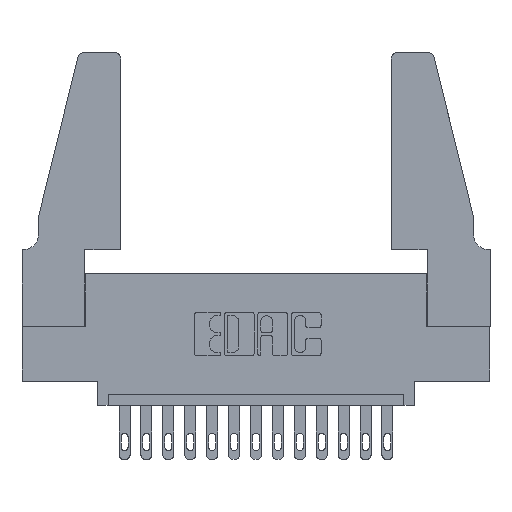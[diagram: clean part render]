
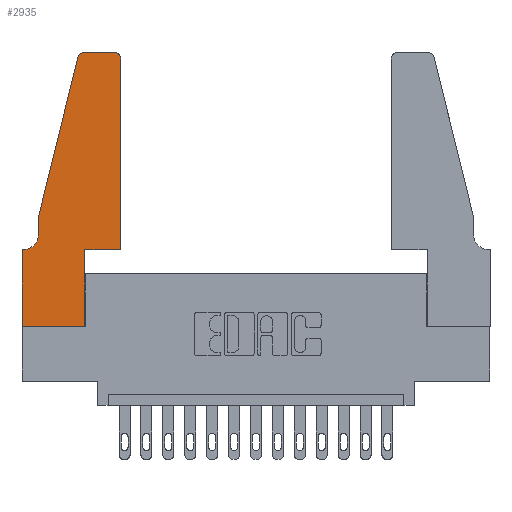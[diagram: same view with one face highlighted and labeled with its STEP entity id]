
A CAD part, top view. The second image highlights one B-rep face of the part: STEP entity #2935.
In plain terms, the highlighted planar face has unit normal (0, 0, 1).
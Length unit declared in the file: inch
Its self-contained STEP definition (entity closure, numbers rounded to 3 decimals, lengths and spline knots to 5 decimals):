
#66 = EDGE_CURVE ( 'NONE', #4315, #12217, #4490, .T. ) ;
#152 = CIRCLE ( 'NONE', #7703, 0.03 ) ;
#831 = CARTESIAN_POINT ( 'NONE',  ( 0.4505, 0.35, 0.37 ) ) ;
#885 = CARTESIAN_POINT ( 'NONE',  ( 0.0055, 0.42, 0.37 ) ) ;
#917 = EDGE_CURVE ( 'NONE', #12802, #11166, #6914, .T. ) ;
#943 = LINE ( 'NONE', #15656, #7222 ) ;
#964 = FACE_OUTER_BOUND ( 'NONE', #8152, .T. ) ;
#1023 = LINE ( 'NONE', #14323, #2944 ) ;
#1383 = CARTESIAN_POINT ( 'NONE',  ( 0.2865, 0., 0.37 ) ) ;
#1442 = CARTESIAN_POINT ( 'NONE',  ( 0.2865, 0.35, 0.37 ) ) ;
#1446 = VERTEX_POINT ( 'NONE', #4714 ) ;
#1695 = CARTESIAN_POINT ( 'NONE',  ( 0.0755, 0.35, 0.37 ) ) ;
#1713 = CARTESIAN_POINT ( 'NONE',  ( 0.0755, 0.5, 0.37 ) ) ;
#2155 = DIRECTION ( 'NONE',  ( 1., 0., 0. ) ) ;
#2235 = ORIENTED_EDGE ( 'NONE', *, *, #4029, .T. ) ;
#2286 = VECTOR ( 'NONE', #13903, 39.37008 ) ;
#2416 = ORIENTED_EDGE ( 'NONE', *, *, #11070, .T. ) ;
#2515 = CARTESIAN_POINT ( 'NONE',  ( 0.4505, 0.35, 0.37 ) ) ;
#2835 = VERTEX_POINT ( 'NONE', #6938 ) ;
#2844 = LINE ( 'NONE', #2515, #15338 ) ;
#2935 = ADVANCED_FACE ( 'NONE', ( #964 ), #7052, .T. ) ;
#2944 = VECTOR ( 'NONE', #10096, 39.37008 ) ;
#3166 = EDGE_CURVE ( 'NONE', #11661, #12802, #12251, .T. ) ;
#3444 = DIRECTION ( 'NONE',  ( 1., 0., 0. ) ) ;
#3966 = ORIENTED_EDGE ( 'NONE', *, *, #8165, .T. ) ;
#4029 = EDGE_CURVE ( 'NONE', #1446, #11661, #152, .T. ) ;
#4234 = DIRECTION ( 'NONE',  ( 0., -1., 0. ) ) ;
#4315 = VERTEX_POINT ( 'NONE', #15828 ) ;
#4490 = LINE ( 'NONE', #1695, #7522 ) ;
#4604 = VECTOR ( 'NONE', #14760, 39.37008 ) ;
#4714 = CARTESIAN_POINT ( 'NONE',  ( 0.4505, 1.22, 0.37 ) ) ;
#4883 = LINE ( 'NONE', #831, #9477 ) ;
#5033 = EDGE_CURVE ( 'NONE', #9683, #4315, #11062, .T. ) ;
#5145 = ORIENTED_EDGE ( 'NONE', *, *, #9306, .T. ) ;
#5272 = ORIENTED_EDGE ( 'NONE', *, *, #5033, .T. ) ;
#5331 = LINE ( 'NONE', #8982, #2286 ) ;
#5389 = ORIENTED_EDGE ( 'NONE', *, *, #66, .T. ) ;
#6042 = CARTESIAN_POINT ( 'NONE',  ( 0.4205, 1.22, 0.37 ) ) ;
#6242 = CARTESIAN_POINT ( 'NONE',  ( 0., 0., 0.37 ) ) ;
#6305 = ORIENTED_EDGE ( 'NONE', *, *, #8051, .T. ) ;
#6515 = DIRECTION ( 'NONE',  ( 1., 0., 0. ) ) ;
#6914 = CIRCLE ( 'NONE', #12190, 0.03 ) ;
#6938 = CARTESIAN_POINT ( 'NONE',  ( 0., 0., 0.37 ) ) ;
#7052 = PLANE ( 'NONE',  #7584 ) ;
#7111 = CARTESIAN_POINT ( 'NONE',  ( 0., 0.35, 0.37 ) ) ;
#7222 = VECTOR ( 'NONE', #4234, 39.37008 ) ;
#7522 = VECTOR ( 'NONE', #12796, 39.37008 ) ;
#7526 = EDGE_CURVE ( 'NONE', #2835, #10246, #10563, .T. ) ;
#7584 = AXIS2_PLACEMENT_3D ( 'NONE', #7111, #8141, #3444 ) ;
#7646 = EDGE_CURVE ( 'NONE', #10246, #10263, #5331, .T. ) ;
#7703 = AXIS2_PLACEMENT_3D ( 'NONE', #6042, #12357, #6515 ) ;
#8051 = EDGE_CURVE ( 'NONE', #12217, #2835, #943, .T. ) ;
#8141 = DIRECTION ( 'NONE',  ( 0., 0., 1. ) ) ;
#8152 = EDGE_LOOP ( 'NONE', ( #9585, #10078, #5145, #9146, #5272, #5389, #6305, #11058, #9573, #2416, #3966, #2235 ) ) ;
#8165 = EDGE_CURVE ( 'NONE', #8953, #1446, #2844, .T. ) ;
#8284 = DIRECTION ( 'NONE',  ( -0.239, -0.971, 0. ) ) ;
#8731 = CARTESIAN_POINT ( 'NONE',  ( 0.25487, 1.22718, 0.37 ) ) ;
#8922 = AXIS2_PLACEMENT_3D ( 'NONE', #885, #12017, #10703 ) ;
#8953 = VERTEX_POINT ( 'NONE', #11876 ) ;
#8982 = CARTESIAN_POINT ( 'NONE',  ( 0.2865, 0.35, 0.37 ) ) ;
#9146 = ORIENTED_EDGE ( 'NONE', *, *, #11663, .T. ) ;
#9306 = EDGE_CURVE ( 'NONE', #11166, #13783, #9516, .T. ) ;
#9477 = VECTOR ( 'NONE', #2155, 39.37008 ) ;
#9516 = LINE ( 'NONE', #9657, #15683 ) ;
#9573 = ORIENTED_EDGE ( 'NONE', *, *, #7646, .T. ) ;
#9585 = ORIENTED_EDGE ( 'NONE', *, *, #3166, .T. ) ;
#9657 = CARTESIAN_POINT ( 'NONE',  ( 0.0755, 0.5, 0.37 ) ) ;
#9683 = VERTEX_POINT ( 'NONE', #9718 ) ;
#9718 = CARTESIAN_POINT ( 'NONE',  ( 0.0755, 0.42, 0.37 ) ) ;
#9745 = CARTESIAN_POINT ( 'NONE',  ( 0.2605, 1.25, 0.37 ) ) ;
#10028 = DIRECTION ( 'NONE',  ( 0., 1., 0. ) ) ;
#10078 = ORIENTED_EDGE ( 'NONE', *, *, #917, .T. ) ;
#10096 = DIRECTION ( 'NONE',  ( 0., -1., 0. ) ) ;
#10246 = VERTEX_POINT ( 'NONE', #1383 ) ;
#10263 = VERTEX_POINT ( 'NONE', #1442 ) ;
#10563 = LINE ( 'NONE', #6242, #4604 ) ;
#10703 = DIRECTION ( 'NONE',  ( -1., 0., 0. ) ) ;
#11058 = ORIENTED_EDGE ( 'NONE', *, *, #7526, .T. ) ;
#11062 = CIRCLE ( 'NONE', #8922, 0.07 ) ;
#11070 = EDGE_CURVE ( 'NONE', #10263, #8953, #4883, .T. ) ;
#11166 = VERTEX_POINT ( 'NONE', #8731 ) ;
#11383 = CARTESIAN_POINT ( 'NONE',  ( 0.4205, 1.25, 0.37 ) ) ;
#11661 = VERTEX_POINT ( 'NONE', #11383 ) ;
#11663 = EDGE_CURVE ( 'NONE', #13783, #9683, #1023, .T. ) ;
#11876 = CARTESIAN_POINT ( 'NONE',  ( 0.4505, 0.35, 0.37 ) ) ;
#12017 = DIRECTION ( 'NONE',  ( 0., 0., -1. ) ) ;
#12103 = CARTESIAN_POINT ( 'NONE',  ( 0.284, 1.25, 0.37 ) ) ;
#12162 = DIRECTION ( 'NONE',  ( 1., 0., 0. ) ) ;
#12190 = AXIS2_PLACEMENT_3D ( 'NONE', #15903, #12524, #12162 ) ;
#12217 = VERTEX_POINT ( 'NONE', #12837 ) ;
#12251 = LINE ( 'NONE', #9745, #13824 ) ;
#12357 = DIRECTION ( 'NONE',  ( 0., 0., 1. ) ) ;
#12524 = DIRECTION ( 'NONE',  ( 0., 0., 1. ) ) ;
#12796 = DIRECTION ( 'NONE',  ( -1., 0., 0. ) ) ;
#12802 = VERTEX_POINT ( 'NONE', #12103 ) ;
#12837 = CARTESIAN_POINT ( 'NONE',  ( 0., 0.35, 0.37 ) ) ;
#13783 = VERTEX_POINT ( 'NONE', #1713 ) ;
#13824 = VECTOR ( 'NONE', #14522, 39.37008 ) ;
#13903 = DIRECTION ( 'NONE',  ( 0., 1., 0. ) ) ;
#14323 = CARTESIAN_POINT ( 'NONE',  ( 0.0755, 0.5, 0.37 ) ) ;
#14522 = DIRECTION ( 'NONE',  ( -1., 0., 0. ) ) ;
#14760 = DIRECTION ( 'NONE',  ( 1., 0., 0. ) ) ;
#15338 = VECTOR ( 'NONE', #10028, 39.37008 ) ;
#15656 = CARTESIAN_POINT ( 'NONE',  ( 0., 0., 0.37 ) ) ;
#15683 = VECTOR ( 'NONE', #8284, 39.37008 ) ;
#15828 = CARTESIAN_POINT ( 'NONE',  ( 0.0055, 0.35, 0.37 ) ) ;
#15903 = CARTESIAN_POINT ( 'NONE',  ( 0.284, 1.22, 0.37 ) ) ;
